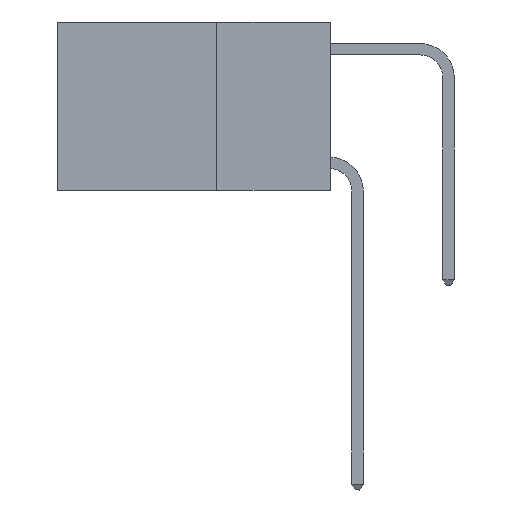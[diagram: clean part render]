
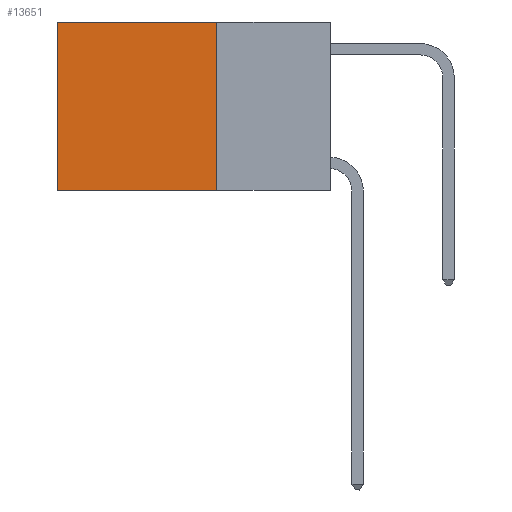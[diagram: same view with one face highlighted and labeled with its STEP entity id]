
A CAD part, left-side view. The second image highlights one B-rep face of the part: STEP entity #13651.
In plain terms, the highlighted planar face has unit normal (-1, 0, 0).
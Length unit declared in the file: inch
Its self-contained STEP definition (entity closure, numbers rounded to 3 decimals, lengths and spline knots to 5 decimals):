
#143 = VECTOR ( 'NONE', #5182, 39.37008 ) ;
#193 = EDGE_LOOP ( 'NONE', ( #9163, #12567, #8675, #6631 ) ) ;
#595 = CARTESIAN_POINT ( 'NONE',  ( 0.2625, 0.25, 0. ) ) ;
#1511 = CARTESIAN_POINT ( 'NONE',  ( 0.2625, 0.25, -0.37 ) ) ;
#1796 = EDGE_CURVE ( 'NONE', #9448, #10328, #4182, .T. ) ;
#2772 = EDGE_CURVE ( 'NONE', #11197, #10328, #3389, .T. ) ;
#2825 = VECTOR ( 'NONE', #4389, 39.37008 ) ;
#3048 = EDGE_CURVE ( 'NONE', #8980, #11197, #9181, .T. ) ;
#3389 = LINE ( 'NONE', #1511, #143 ) ;
#4182 = LINE ( 'NONE', #13818, #7750 ) ;
#4297 = AXIS2_PLACEMENT_3D ( 'NONE', #11425, #6744, #14920 ) ;
#4389 = DIRECTION ( 'NONE',  ( 0., 0., -1. ) ) ;
#4424 = CARTESIAN_POINT ( 'NONE',  ( 0.2625, 0.25, -0.37 ) ) ;
#5182 = DIRECTION ( 'NONE',  ( 0., 1., 0. ) ) ;
#6631 = ORIENTED_EDGE ( 'NONE', *, *, #14811, .T. ) ;
#6691 = PLANE ( 'NONE',  #4297 ) ;
#6744 = DIRECTION ( 'NONE',  ( 1., 0., 0. ) ) ;
#7750 = VECTOR ( 'NONE', #7989, 39.37008 ) ;
#7989 = DIRECTION ( 'NONE',  ( 0., 0., -1. ) ) ;
#8675 = ORIENTED_EDGE ( 'NONE', *, *, #3048, .F. ) ;
#8953 = CARTESIAN_POINT ( 'NONE',  ( 0.2625, 0.6, 0. ) ) ;
#8980 = VERTEX_POINT ( 'NONE', #595 ) ;
#9163 = ORIENTED_EDGE ( 'NONE', *, *, #1796, .T. ) ;
#9181 = LINE ( 'NONE', #12685, #2825 ) ;
#9448 = VERTEX_POINT ( 'NONE', #8953 ) ;
#10328 = VERTEX_POINT ( 'NONE', #12285 ) ;
#10390 = FACE_OUTER_BOUND ( 'NONE', #193, .T. ) ;
#11197 = VERTEX_POINT ( 'NONE', #4424 ) ;
#11425 = CARTESIAN_POINT ( 'NONE',  ( 0.2625, 0.25, 0. ) ) ;
#12285 = CARTESIAN_POINT ( 'NONE',  ( 0.2625, 0.6, -0.37 ) ) ;
#12414 = LINE ( 'NONE', #12583, #15091 ) ;
#12567 = ORIENTED_EDGE ( 'NONE', *, *, #2772, .F. ) ;
#12583 = CARTESIAN_POINT ( 'NONE',  ( 0.2625, 0.25, 0. ) ) ;
#12685 = CARTESIAN_POINT ( 'NONE',  ( 0.2625, 0.25, 0. ) ) ;
#13651 = ADVANCED_FACE ( 'NONE', ( #10390 ), #6691, .F. ) ;
#13734 = DIRECTION ( 'NONE',  ( 0., 1., 0. ) ) ;
#13818 = CARTESIAN_POINT ( 'NONE',  ( 0.2625, 0.6, 0. ) ) ;
#14811 = EDGE_CURVE ( 'NONE', #8980, #9448, #12414, .T. ) ;
#14920 = DIRECTION ( 'NONE',  ( 0., 0., -1. ) ) ;
#15091 = VECTOR ( 'NONE', #13734, 39.37008 ) ;
